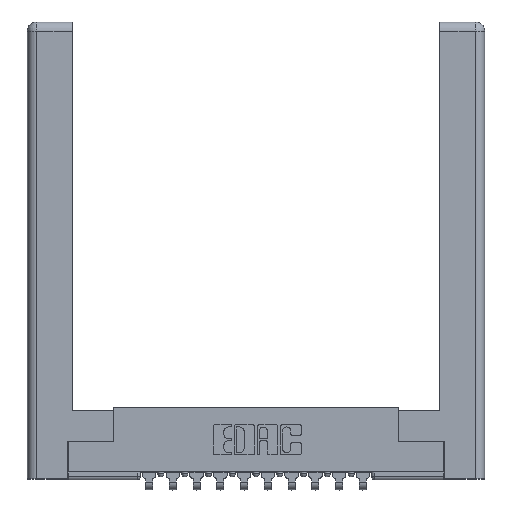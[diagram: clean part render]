
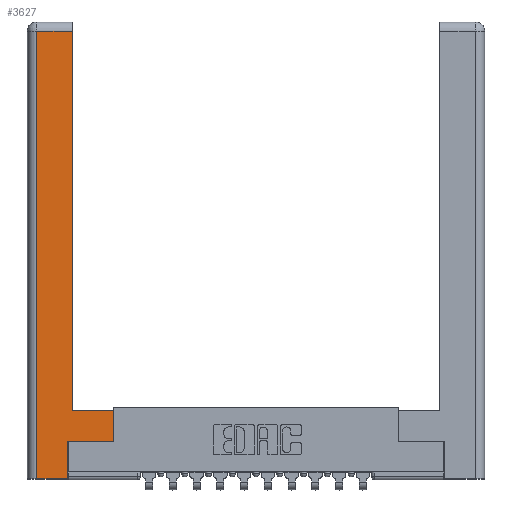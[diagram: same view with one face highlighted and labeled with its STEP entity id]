
A CAD part, top view. The second image highlights one B-rep face of the part: STEP entity #3627.
In plain terms, the highlighted planar face has unit normal (0, 0, 1).
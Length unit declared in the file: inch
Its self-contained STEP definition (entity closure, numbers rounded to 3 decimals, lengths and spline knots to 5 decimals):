
#237 = AXIS2_PLACEMENT_3D ( 'NONE', #6820, #2028, #422 ) ;
#422 = DIRECTION ( 'NONE',  ( -1., 0., 0. ) ) ;
#741 = LINE ( 'NONE', #11250, #7500 ) ;
#810 = VECTOR ( 'NONE', #6501, 39.37008 ) ;
#1155 = LINE ( 'NONE', #7274, #11142 ) ;
#1237 = DIRECTION ( 'NONE',  ( -1., 0., 0. ) ) ;
#1488 = LINE ( 'NONE', #1772, #810 ) ;
#1628 = VERTEX_POINT ( 'NONE', #11498 ) ;
#1772 = CARTESIAN_POINT ( 'NONE',  ( 0.0615, 2.94, 0. ) ) ;
#1798 = ORIENTED_EDGE ( 'NONE', *, *, #13494, .T. ) ;
#1844 = CARTESIAN_POINT ( 'NONE',  ( 0.295, 2.94, 0. ) ) ;
#1961 = DIRECTION ( 'NONE',  ( 0., -1., 0. ) ) ;
#2028 = DIRECTION ( 'NONE',  ( 0., 0., -1. ) ) ;
#2050 = DIRECTION ( 'NONE',  ( 0., 1., 0. ) ) ;
#2391 = LINE ( 'NONE', #11821, #8265 ) ;
#2408 = DIRECTION ( 'NONE',  ( 1., 0., 0. ) ) ;
#2676 = VERTEX_POINT ( 'NONE', #3932 ) ;
#2955 = FACE_OUTER_BOUND ( 'NONE', #9421, .T. ) ;
#3305 = CARTESIAN_POINT ( 'NONE',  ( 0.565, 0.45, 0. ) ) ;
#3627 = ADVANCED_FACE ( 'NONE', ( #2955 ), #7699, .F. ) ;
#3654 = EDGE_CURVE ( 'NONE', #14476, #13058, #3962, .T. ) ;
#3932 = CARTESIAN_POINT ( 'NONE',  ( 0.265, 0., 0. ) ) ;
#3962 = LINE ( 'NONE', #5665, #10136 ) ;
#4588 = LINE ( 'NONE', #9479, #15229 ) ;
#4723 = VERTEX_POINT ( 'NONE', #14096 ) ;
#4729 = ORIENTED_EDGE ( 'NONE', *, *, #9735, .T. ) ;
#5278 = VERTEX_POINT ( 'NONE', #9150 ) ;
#5665 = CARTESIAN_POINT ( 'NONE',  ( 0.565, 0.45, 0. ) ) ;
#5976 = CARTESIAN_POINT ( 'NONE',  ( 0.265, 0., 0. ) ) ;
#6501 = DIRECTION ( 'NONE',  ( -1., 0., 0. ) ) ;
#6820 = CARTESIAN_POINT ( 'NONE',  ( 0., 0., 0. ) ) ;
#6926 = CARTESIAN_POINT ( 'NONE',  ( 0.565, 0.245, 0. ) ) ;
#7158 = EDGE_CURVE ( 'NONE', #2676, #11284, #4588, .T. ) ;
#7274 = CARTESIAN_POINT ( 'NONE',  ( 0.565, 0.245, 0. ) ) ;
#7292 = LINE ( 'NONE', #5976, #14077 ) ;
#7500 = VECTOR ( 'NONE', #11555, 39.37008 ) ;
#7549 = DIRECTION ( 'NONE',  ( 0., 1., 0. ) ) ;
#7699 = PLANE ( 'NONE',  #237 ) ;
#8265 = VECTOR ( 'NONE', #1237, 39.37008 ) ;
#8529 = ORIENTED_EDGE ( 'NONE', *, *, #13683, .T. ) ;
#9083 = CARTESIAN_POINT ( 'NONE',  ( 0.0615, 0., 0. ) ) ;
#9150 = CARTESIAN_POINT ( 'NONE',  ( 0.295, 0.45, 0. ) ) ;
#9421 = EDGE_LOOP ( 'NONE', ( #1798, #13583, #11855, #4729, #10349, #10401, #9541, #8529 ) ) ;
#9479 = CARTESIAN_POINT ( 'NONE',  ( 0.265, 0.245, 0. ) ) ;
#9541 = ORIENTED_EDGE ( 'NONE', *, *, #3654, .T. ) ;
#9735 = EDGE_CURVE ( 'NONE', #1628, #2676, #7292, .T. ) ;
#10073 = EDGE_CURVE ( 'NONE', #11284, #14476, #1155, .T. ) ;
#10136 = VECTOR ( 'NONE', #7549, 39.37008 ) ;
#10349 = ORIENTED_EDGE ( 'NONE', *, *, #7158, .T. ) ;
#10401 = ORIENTED_EDGE ( 'NONE', *, *, #10073, .T. ) ;
#11142 = VECTOR ( 'NONE', #12823, 39.37008 ) ;
#11250 = CARTESIAN_POINT ( 'NONE',  ( 0.295, 3., 0. ) ) ;
#11284 = VERTEX_POINT ( 'NONE', #12672 ) ;
#11498 = CARTESIAN_POINT ( 'NONE',  ( 0.0615, 0., 0. ) ) ;
#11555 = DIRECTION ( 'NONE',  ( 0., 1., 0. ) ) ;
#11812 = VERTEX_POINT ( 'NONE', #1844 ) ;
#11821 = CARTESIAN_POINT ( 'NONE',  ( 0.295, 0.45, 0. ) ) ;
#11855 = ORIENTED_EDGE ( 'NONE', *, *, #14760, .T. ) ;
#12383 = LINE ( 'NONE', #9083, #13189 ) ;
#12672 = CARTESIAN_POINT ( 'NONE',  ( 0.265, 0.245, 0. ) ) ;
#12823 = DIRECTION ( 'NONE',  ( 1., 0., 0. ) ) ;
#12980 = EDGE_CURVE ( 'NONE', #11812, #4723, #1488, .T. ) ;
#13058 = VERTEX_POINT ( 'NONE', #3305 ) ;
#13189 = VECTOR ( 'NONE', #1961, 39.37008 ) ;
#13494 = EDGE_CURVE ( 'NONE', #5278, #11812, #741, .T. ) ;
#13583 = ORIENTED_EDGE ( 'NONE', *, *, #12980, .T. ) ;
#13683 = EDGE_CURVE ( 'NONE', #13058, #5278, #2391, .T. ) ;
#14077 = VECTOR ( 'NONE', #2408, 39.37008 ) ;
#14096 = CARTESIAN_POINT ( 'NONE',  ( 0.0615, 2.94, 0. ) ) ;
#14476 = VERTEX_POINT ( 'NONE', #6926 ) ;
#14760 = EDGE_CURVE ( 'NONE', #4723, #1628, #12383, .T. ) ;
#15229 = VECTOR ( 'NONE', #2050, 39.37008 ) ;
